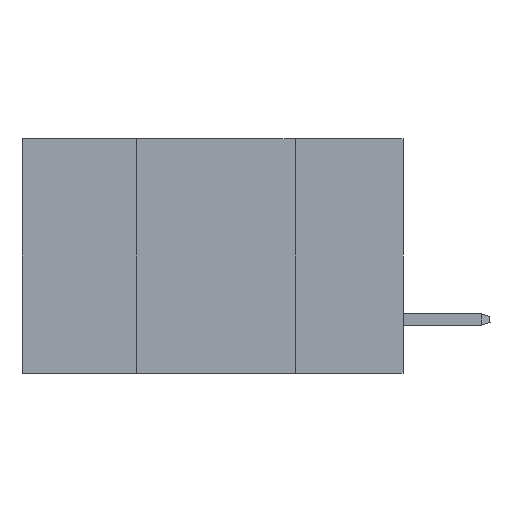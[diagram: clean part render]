
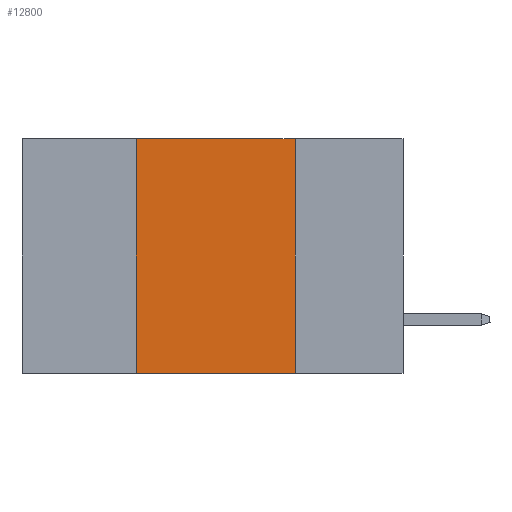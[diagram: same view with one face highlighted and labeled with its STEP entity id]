
A CAD part, left-side view. The second image highlights one B-rep face of the part: STEP entity #12800.
In plain terms, the highlighted planar face has unit normal (-1, 0, 0).
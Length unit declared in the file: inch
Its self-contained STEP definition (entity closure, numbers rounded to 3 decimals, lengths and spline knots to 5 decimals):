
#65 = FACE_OUTER_BOUND ( 'NONE', #560, .T. ) ;
#560 = EDGE_LOOP ( 'NONE', ( #9916, #4274, #14717, #14026 ) ) ;
#796 = EDGE_CURVE ( 'NONE', #5981, #3166, #3612, .T. ) ;
#1423 = PLANE ( 'NONE',  #12410 ) ;
#2789 = DIRECTION ( 'NONE',  ( 0., -1., 0. ) ) ;
#2841 = DIRECTION ( 'NONE',  ( 1., 0., 0. ) ) ;
#3166 = VERTEX_POINT ( 'NONE', #8458 ) ;
#3308 = DIRECTION ( 'NONE',  ( 0., 0., 1. ) ) ;
#3612 = LINE ( 'NONE', #10232, #17109 ) ;
#3626 = EDGE_CURVE ( 'NONE', #11602, #5981, #8311, .T. ) ;
#4123 = CARTESIAN_POINT ( 'NONE',  ( 0., 0.6, 0. ) ) ;
#4274 = ORIENTED_EDGE ( 'NONE', *, *, #3626, .F. ) ;
#5764 = VERTEX_POINT ( 'NONE', #15753 ) ;
#5981 = VERTEX_POINT ( 'NONE', #17515 ) ;
#6151 = CARTESIAN_POINT ( 'NONE',  ( 0., 0.6, -0.37 ) ) ;
#6387 = VECTOR ( 'NONE', #2789, 39.37008 ) ;
#7839 = EDGE_CURVE ( 'NONE', #5764, #3166, #15498, .T. ) ;
#8311 = LINE ( 'NONE', #4123, #6387 ) ;
#8458 = CARTESIAN_POINT ( 'NONE',  ( 0., 0.17, -0.37 ) ) ;
#9626 = CARTESIAN_POINT ( 'NONE',  ( 0., 0.6, 0. ) ) ;
#9916 = ORIENTED_EDGE ( 'NONE', *, *, #796, .F. ) ;
#10224 = CARTESIAN_POINT ( 'NONE',  ( 0., 0.42, 0. ) ) ;
#10232 = CARTESIAN_POINT ( 'NONE',  ( 0., 0.17, 0. ) ) ;
#10707 = VECTOR ( 'NONE', #13096, 39.37008 ) ;
#11602 = VERTEX_POINT ( 'NONE', #10224 ) ;
#12410 = AXIS2_PLACEMENT_3D ( 'NONE', #9626, #2841, #17538 ) ;
#12800 = ADVANCED_FACE ( 'NONE', ( #65 ), #1423, .F. ) ;
#13096 = DIRECTION ( 'NONE',  ( 0., -1., 0. ) ) ;
#13808 = EDGE_CURVE ( 'NONE', #5764, #11602, #13926, .T. ) ;
#13926 = LINE ( 'NONE', #15515, #16930 ) ;
#14026 = ORIENTED_EDGE ( 'NONE', *, *, #7839, .T. ) ;
#14717 = ORIENTED_EDGE ( 'NONE', *, *, #13808, .F. ) ;
#15498 = LINE ( 'NONE', #6151, #10707 ) ;
#15515 = CARTESIAN_POINT ( 'NONE',  ( 0., 0.42, 0. ) ) ;
#15733 = DIRECTION ( 'NONE',  ( 0., 0., -1. ) ) ;
#15753 = CARTESIAN_POINT ( 'NONE',  ( 0., 0.42, -0.37 ) ) ;
#16930 = VECTOR ( 'NONE', #3308, 39.37008 ) ;
#17109 = VECTOR ( 'NONE', #15733, 39.37008 ) ;
#17515 = CARTESIAN_POINT ( 'NONE',  ( 0., 0.17, 0. ) ) ;
#17538 = DIRECTION ( 'NONE',  ( 0., 0., -1. ) ) ;
